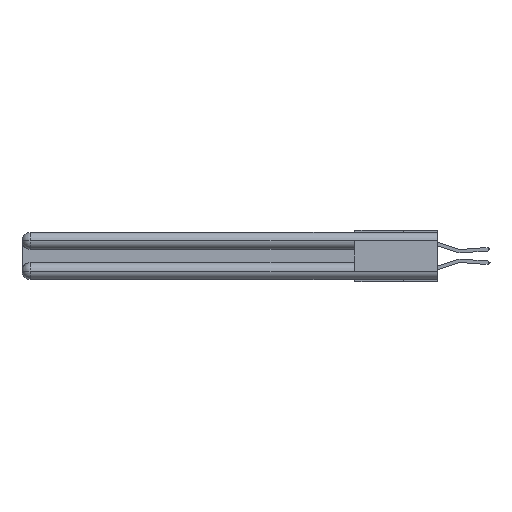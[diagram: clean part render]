
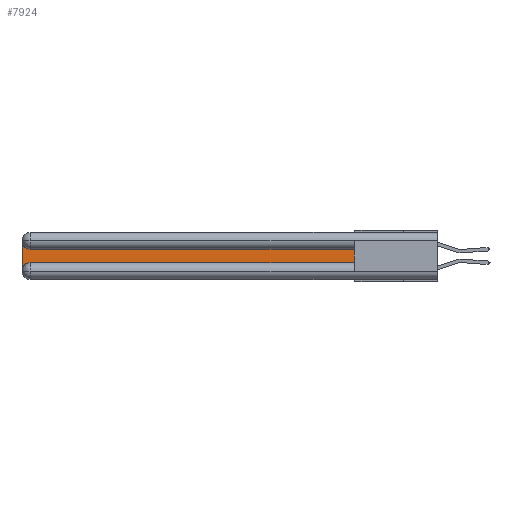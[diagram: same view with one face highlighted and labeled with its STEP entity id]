
A CAD part, left-side view. The second image highlights one B-rep face of the part: STEP entity #7924.
In plain terms, the highlighted planar face has unit normal (-1, 0, 0).
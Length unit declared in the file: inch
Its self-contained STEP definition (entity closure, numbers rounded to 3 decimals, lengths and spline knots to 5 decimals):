
#940 = EDGE_CURVE ( 'NONE', #6915, #2195, #1093, .T. ) ;
#1093 = LINE ( 'NONE', #19163, #2794 ) ;
#1884 = VERTEX_POINT ( 'NONE', #3912 ) ;
#2185 = EDGE_CURVE ( 'NONE', #13982, #1884, #28335, .T. ) ;
#2195 = VERTEX_POINT ( 'NONE', #8782 ) ;
#2461 = EDGE_CURVE ( 'NONE', #2195, #28790, #16791, .T. ) ;
#2794 = VECTOR ( 'NONE', #5974, 39.37008 ) ;
#3912 = CARTESIAN_POINT ( 'NONE',  ( 0.075, 0.6, -0.1225 ) ) ;
#4050 = VECTOR ( 'NONE', #5992, 39.37008 ) ;
#4223 = CARTESIAN_POINT ( 'NONE',  ( 0.075, 0.6, -0.2175 ) ) ;
#4792 = CARTESIAN_POINT ( 'NONE',  ( 0.075, 2.94, -0.2775 ) ) ;
#5974 = DIRECTION ( 'NONE',  ( 0., 0., -1. ) ) ;
#5992 = DIRECTION ( 'NONE',  ( 0., 0., 1. ) ) ;
#6405 = LINE ( 'NONE', #12320, #8988 ) ;
#6861 = CARTESIAN_POINT ( 'NONE',  ( 0.075, 3., -0.0625 ) ) ;
#6915 = VERTEX_POINT ( 'NONE', #6861 ) ;
#7619 = ORIENTED_EDGE ( 'NONE', *, *, #940, .T. ) ;
#7924 = ADVANCED_FACE ( 'NONE', ( #27137 ), #33977, .F. ) ;
#8451 = ORIENTED_EDGE ( 'NONE', *, *, #32837, .T. ) ;
#8782 = CARTESIAN_POINT ( 'NONE',  ( 0.075, 3., -0.2775 ) ) ;
#8955 = VECTOR ( 'NONE', #27411, 39.37008 ) ;
#8988 = VECTOR ( 'NONE', #14798, 39.37008 ) ;
#9082 = DIRECTION ( 'NONE',  ( 1., 0., 0. ) ) ;
#11847 = CARTESIAN_POINT ( 'NONE',  ( 0.075, 2.94, -0.0625 ) ) ;
#12056 = ORIENTED_EDGE ( 'NONE', *, *, #32455, .T. ) ;
#12320 = CARTESIAN_POINT ( 'NONE',  ( 0.075, 0.6, -0.1225 ) ) ;
#12403 = AXIS2_PLACEMENT_3D ( 'NONE', #4792, #29207, #26565 ) ;
#12691 = CIRCLE ( 'NONE', #25008, 0.06 ) ;
#13143 = ORIENTED_EDGE ( 'NONE', *, *, #2461, .T. ) ;
#13982 = VERTEX_POINT ( 'NONE', #4223 ) ;
#14100 = CARTESIAN_POINT ( 'NONE',  ( 0.075, 0.6, -0.2175 ) ) ;
#14675 = DIRECTION ( 'NONE',  ( 0., 0., -1. ) ) ;
#14719 = EDGE_LOOP ( 'NONE', ( #12056, #35188, #7619, #13143, #8451, #33535 ) ) ;
#14798 = DIRECTION ( 'NONE',  ( 0., 1., 0. ) ) ;
#14980 = VERTEX_POINT ( 'NONE', #21569 ) ;
#16791 = CIRCLE ( 'NONE', #12403, 0.06 ) ;
#17525 = EDGE_CURVE ( 'NONE', #14980, #6915, #12691, .T. ) ;
#19163 = CARTESIAN_POINT ( 'NONE',  ( 0.075, 3., -0.2175 ) ) ;
#21569 = CARTESIAN_POINT ( 'NONE',  ( 0.075, 2.94, -0.1225 ) ) ;
#21876 = CARTESIAN_POINT ( 'NONE',  ( 0.075, 0.6, -0.2175 ) ) ;
#24369 = AXIS2_PLACEMENT_3D ( 'NONE', #25848, #9082, #28357 ) ;
#25008 = AXIS2_PLACEMENT_3D ( 'NONE', #11847, #33688, #14675 ) ;
#25848 = CARTESIAN_POINT ( 'NONE',  ( 0.075, 3., -0.1225 ) ) ;
#26400 = LINE ( 'NONE', #21876, #8955 ) ;
#26565 = DIRECTION ( 'NONE',  ( 0., 0., -1. ) ) ;
#27137 = FACE_OUTER_BOUND ( 'NONE', #14719, .T. ) ;
#27411 = DIRECTION ( 'NONE',  ( 0., -1., 0. ) ) ;
#28335 = LINE ( 'NONE', #14100, #4050 ) ;
#28357 = DIRECTION ( 'NONE',  ( 0., 0., -1. ) ) ;
#28790 = VERTEX_POINT ( 'NONE', #29832 ) ;
#29207 = DIRECTION ( 'NONE',  ( 1., 0., 0. ) ) ;
#29832 = CARTESIAN_POINT ( 'NONE',  ( 0.075, 2.94, -0.2175 ) ) ;
#32455 = EDGE_CURVE ( 'NONE', #1884, #14980, #6405, .T. ) ;
#32837 = EDGE_CURVE ( 'NONE', #28790, #13982, #26400, .T. ) ;
#33535 = ORIENTED_EDGE ( 'NONE', *, *, #2185, .T. ) ;
#33688 = DIRECTION ( 'NONE',  ( 1., 0., 0. ) ) ;
#33977 = PLANE ( 'NONE',  #24369 ) ;
#35188 = ORIENTED_EDGE ( 'NONE', *, *, #17525, .T. ) ;
